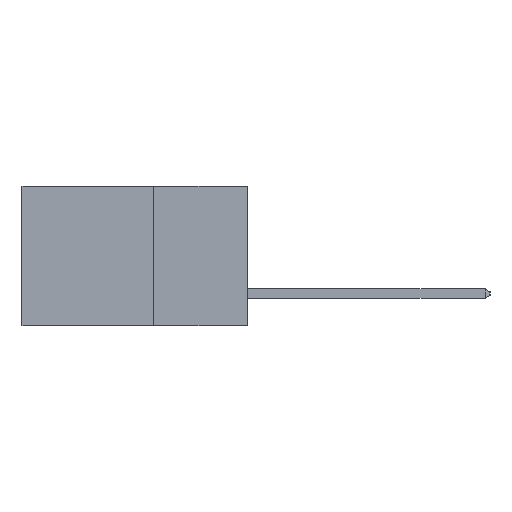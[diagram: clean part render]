
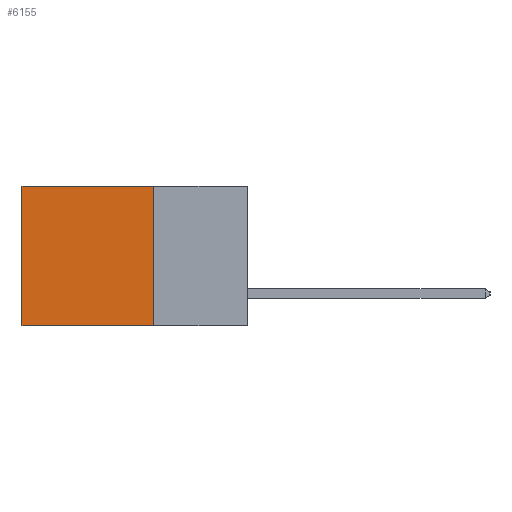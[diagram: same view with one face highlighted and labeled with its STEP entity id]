
A CAD part, left-side view. The second image highlights one B-rep face of the part: STEP entity #6155.
In plain terms, the highlighted planar face has unit normal (-1, 0, 0).
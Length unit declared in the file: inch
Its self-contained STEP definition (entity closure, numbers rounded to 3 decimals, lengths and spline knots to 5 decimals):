
#68 = DIRECTION ( 'NONE',  ( 0., 0., -1. ) ) ;
#81 = CARTESIAN_POINT ( 'NONE',  ( 0.2615, 0.6, -0.37 ) ) ;
#1016 = AXIS2_PLACEMENT_3D ( 'NONE', #18117, #17928, #17861 ) ;
#1172 = EDGE_LOOP ( 'NONE', ( #8672, #17767, #7634, #14116 ) ) ;
#2380 = VECTOR ( 'NONE', #68, 39.37008 ) ;
#2470 = VERTEX_POINT ( 'NONE', #3463 ) ;
#3085 = CARTESIAN_POINT ( 'NONE',  ( 0.2615, 0.25, -0.37 ) ) ;
#3406 = LINE ( 'NONE', #14621, #11628 ) ;
#3449 = DIRECTION ( 'NONE',  ( 0., 1., 0. ) ) ;
#3463 = CARTESIAN_POINT ( 'NONE',  ( 0.2615, 0.6, 0. ) ) ;
#4429 = FACE_OUTER_BOUND ( 'NONE', #1172, .T. ) ;
#4939 = EDGE_CURVE ( 'NONE', #2470, #11805, #14958, .T. ) ;
#4941 = CARTESIAN_POINT ( 'NONE',  ( 0.2615, 0.25, 0. ) ) ;
#6155 = ADVANCED_FACE ( 'NONE', ( #4429 ), #18072, .F. ) ;
#6560 = EDGE_CURVE ( 'NONE', #14385, #11473, #15336, .T. ) ;
#7488 = EDGE_CURVE ( 'NONE', #11473, #11805, #13290, .T. ) ;
#7634 = ORIENTED_EDGE ( 'NONE', *, *, #6560, .F. ) ;
#8672 = ORIENTED_EDGE ( 'NONE', *, *, #4939, .T. ) ;
#8951 = VECTOR ( 'NONE', #3449, 39.37008 ) ;
#10982 = CARTESIAN_POINT ( 'NONE',  ( 0.2615, 0.25, -0.37 ) ) ;
#11473 = VERTEX_POINT ( 'NONE', #10982 ) ;
#11628 = VECTOR ( 'NONE', #16198, 39.37008 ) ;
#11805 = VERTEX_POINT ( 'NONE', #15041 ) ;
#13290 = LINE ( 'NONE', #3085, #8951 ) ;
#13503 = DIRECTION ( 'NONE',  ( 0., 0., -1. ) ) ;
#13662 = CARTESIAN_POINT ( 'NONE',  ( 0.2615, 0.25, -0.37 ) ) ;
#14116 = ORIENTED_EDGE ( 'NONE', *, *, #20845, .T. ) ;
#14341 = VECTOR ( 'NONE', #13503, 39.37008 ) ;
#14385 = VERTEX_POINT ( 'NONE', #4941 ) ;
#14621 = CARTESIAN_POINT ( 'NONE',  ( 0.2615, 0.25, 0. ) ) ;
#14958 = LINE ( 'NONE', #81, #2380 ) ;
#15041 = CARTESIAN_POINT ( 'NONE',  ( 0.2615, 0.6, -0.37 ) ) ;
#15336 = LINE ( 'NONE', #13662, #14341 ) ;
#16198 = DIRECTION ( 'NONE',  ( 0., 1., 0. ) ) ;
#17767 = ORIENTED_EDGE ( 'NONE', *, *, #7488, .F. ) ;
#17861 = DIRECTION ( 'NONE',  ( 0., 0., -1. ) ) ;
#17928 = DIRECTION ( 'NONE',  ( 1., 0., 0. ) ) ;
#18072 = PLANE ( 'NONE',  #1016 ) ;
#18117 = CARTESIAN_POINT ( 'NONE',  ( 0.2615, 0.25, -0.37 ) ) ;
#20845 = EDGE_CURVE ( 'NONE', #14385, #2470, #3406, .T. ) ;
